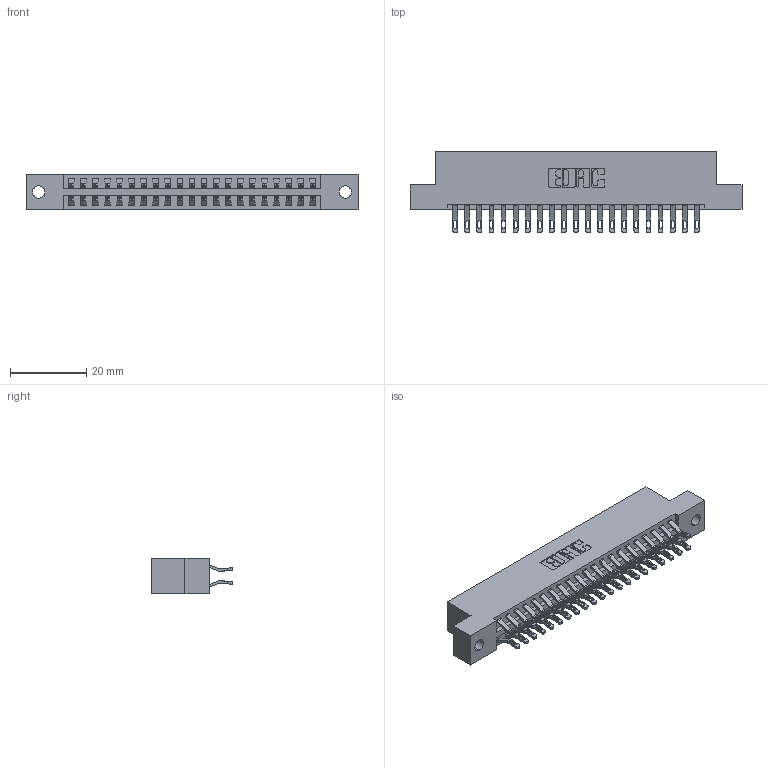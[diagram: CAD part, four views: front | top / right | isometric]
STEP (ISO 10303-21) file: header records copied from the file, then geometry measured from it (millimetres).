
FILE_DESCRIPTION (( 'STEP AP203' ), '1' );
FILE_NAME ('396-042-555-202.STEP', '2019-10-30T11:06:32', ( '' ), ( '' ), 'SwSTEP 2.0', 'SolidWorks 2016', '' );
FILE_SCHEMA (( 'CONFIG_CONTROL_DESIGN' ));
Length unit declared in the file: inch
Products named in the file (3): 396-042-555-202; 346 Part_Flush Mounting Lugs - 0.128 Dia; 345-292-001_555 Tail
Assembly tree (43 placements, depth 2):
  396-042-555-202
    346 Part_Flush Mounting Lugs - 0.128 Dia
    345-292-001_555 Tail  x42
Bounding box: 87.25 x 21.46 x 9.4 mm (x, y, z)
Volume: 8429.9 mm3; surface area: 11422.4 mm2
Topology: 43 solids, 43 shells, 2558 faces, 8015 edges, 5342 vertices
Faces by surface type: plane 1462, cylinder 1096
Entity records: 16861 total; most frequent: CARTESIAN_POINT 2842, ORIENTED_EDGE 2746, DIRECTION 2525, EDGE_CURVE 1373, VECTOR 1137, LINE 1137, VERTEX_POINT 914, AXIS2_PLACEMENT_3D 694
